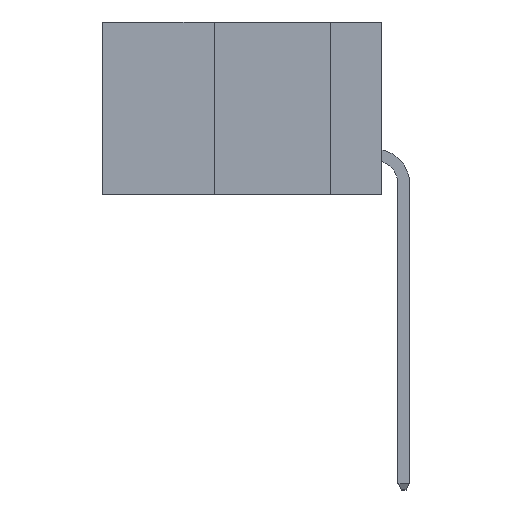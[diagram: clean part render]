
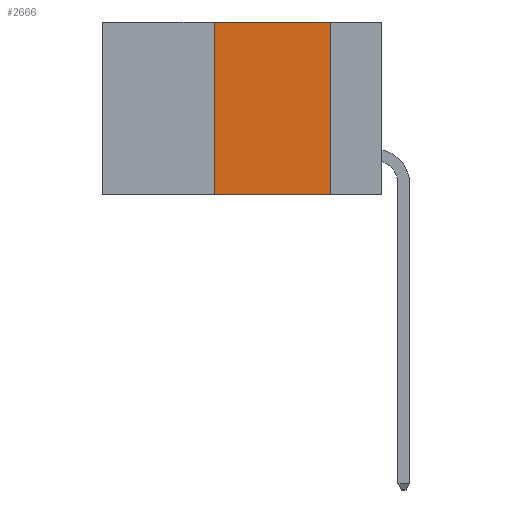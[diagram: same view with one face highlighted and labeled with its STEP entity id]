
A CAD part, left-side view. The second image highlights one B-rep face of the part: STEP entity #2666.
In plain terms, the highlighted planar face has unit normal (-1, 0, 0).
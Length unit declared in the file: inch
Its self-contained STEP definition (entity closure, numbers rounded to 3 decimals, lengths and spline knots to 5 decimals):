
#1248 = LINE ( 'NONE', #29530, #20658 ) ;
#2490 = EDGE_LOOP ( 'NONE', ( #35376, #4167, #19787, #28192 ) ) ;
#2666 = ADVANCED_FACE ( 'NONE', ( #31333 ), #6557, .F. ) ;
#2985 = CARTESIAN_POINT ( 'NONE',  ( 0., 0.11, 0. ) ) ;
#3044 = DIRECTION ( 'NONE',  ( 1., 0., 0. ) ) ;
#4167 = ORIENTED_EDGE ( 'NONE', *, *, #15386, .F. ) ;
#4718 = CARTESIAN_POINT ( 'NONE',  ( 0., 0.36, 0. ) ) ;
#6366 = DIRECTION ( 'NONE',  ( 0., 0., -1. ) ) ;
#6557 = PLANE ( 'NONE',  #20569 ) ;
#11039 = CARTESIAN_POINT ( 'NONE',  ( 0., 0.36, 0. ) ) ;
#13039 = EDGE_CURVE ( 'NONE', #42261, #34254, #1248, .T. ) ;
#13959 = CARTESIAN_POINT ( 'NONE',  ( 0., 0.36, -0.37 ) ) ;
#15204 = DIRECTION ( 'NONE',  ( 0., -1., 0. ) ) ;
#15386 = EDGE_CURVE ( 'NONE', #16476, #29988, #18419, .T. ) ;
#16126 = DIRECTION ( 'NONE',  ( 0., -1., 0. ) ) ;
#16476 = VERTEX_POINT ( 'NONE', #4718 ) ;
#17362 = VECTOR ( 'NONE', #15204, 39.37008 ) ;
#18419 = LINE ( 'NONE', #35360, #17362 ) ;
#19787 = ORIENTED_EDGE ( 'NONE', *, *, #20371, .F. ) ;
#20067 = CARTESIAN_POINT ( 'NONE',  ( 0., 0.11, 0. ) ) ;
#20371 = EDGE_CURVE ( 'NONE', #42261, #16476, #31692, .T. ) ;
#20569 = AXIS2_PLACEMENT_3D ( 'NONE', #23100, #3044, #30065 ) ;
#20658 = VECTOR ( 'NONE', #16126, 39.37008 ) ;
#21297 = DIRECTION ( 'NONE',  ( 0., 0., 1. ) ) ;
#23100 = CARTESIAN_POINT ( 'NONE',  ( 0., 0.6, 0. ) ) ;
#25148 = CARTESIAN_POINT ( 'NONE',  ( 0., 0.11, -0.37 ) ) ;
#28192 = ORIENTED_EDGE ( 'NONE', *, *, #13039, .T. ) ;
#29530 = CARTESIAN_POINT ( 'NONE',  ( 0., 0.6, -0.37 ) ) ;
#29988 = VERTEX_POINT ( 'NONE', #20067 ) ;
#30065 = DIRECTION ( 'NONE',  ( 0., 0., -1. ) ) ;
#30077 = VECTOR ( 'NONE', #6366, 39.37008 ) ;
#31333 = FACE_OUTER_BOUND ( 'NONE', #2490, .T. ) ;
#31692 = LINE ( 'NONE', #11039, #34851 ) ;
#34254 = VERTEX_POINT ( 'NONE', #25148 ) ;
#34851 = VECTOR ( 'NONE', #21297, 39.37008 ) ;
#35360 = CARTESIAN_POINT ( 'NONE',  ( 0., 0.6, 0. ) ) ;
#35376 = ORIENTED_EDGE ( 'NONE', *, *, #40999, .F. ) ;
#40609 = LINE ( 'NONE', #2985, #30077 ) ;
#40999 = EDGE_CURVE ( 'NONE', #29988, #34254, #40609, .T. ) ;
#42261 = VERTEX_POINT ( 'NONE', #13959 ) ;
